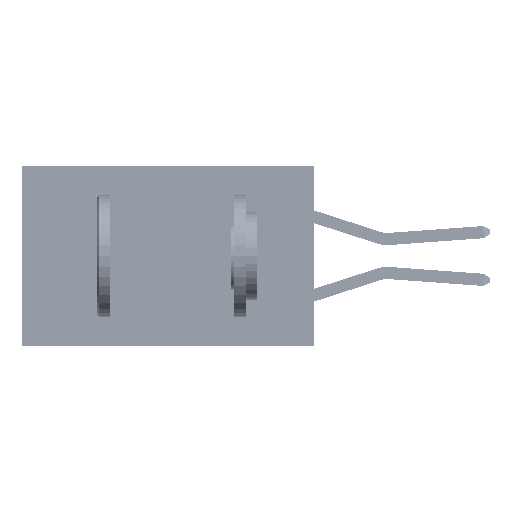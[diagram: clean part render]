
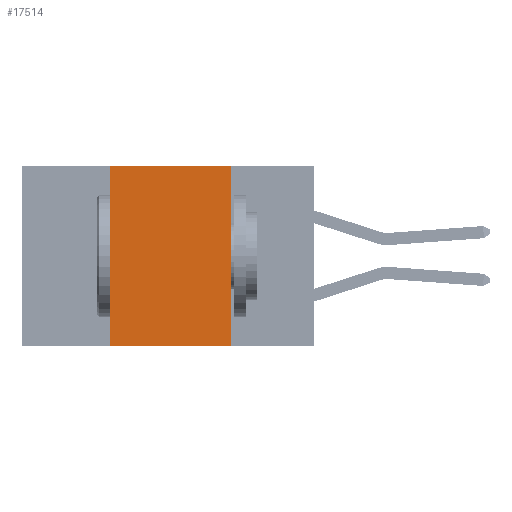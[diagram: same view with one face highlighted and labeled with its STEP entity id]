
A CAD part, left-side view. The second image highlights one B-rep face of the part: STEP entity #17514.
In plain terms, the highlighted planar face has unit normal (-1, 0, 0).
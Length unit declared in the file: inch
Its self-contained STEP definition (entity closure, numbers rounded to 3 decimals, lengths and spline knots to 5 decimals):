
#2994 = VERTEX_POINT ( 'NONE', #39221 ) ;
#3120 = CARTESIAN_POINT ( 'NONE',  ( 0., 0.42, 0. ) ) ;
#3988 = ORIENTED_EDGE ( 'NONE', *, *, #10687, .F. ) ;
#4960 = VERTEX_POINT ( 'NONE', #11925 ) ;
#8691 = EDGE_LOOP ( 'NONE', ( #48236, #26833, #3988, #29303 ) ) ;
#10092 = EDGE_CURVE ( 'NONE', #31452, #2994, #28479, .T. ) ;
#10687 = EDGE_CURVE ( 'NONE', #31452, #4960, #23612, .T. ) ;
#11925 = CARTESIAN_POINT ( 'NONE',  ( 0., 0.42, 0. ) ) ;
#12574 = LINE ( 'NONE', #23094, #21765 ) ;
#13145 = DIRECTION ( 'NONE',  ( 1., 0., 0. ) ) ;
#17514 = ADVANCED_FACE ( 'NONE', ( #49856 ), #32469, .F. ) ;
#18030 = EDGE_CURVE ( 'NONE', #4960, #30088, #28951, .T. ) ;
#18558 = VECTOR ( 'NONE', #28494, 39.37008 ) ;
#18847 = AXIS2_PLACEMENT_3D ( 'NONE', #36596, #13145, #40510 ) ;
#19148 = DIRECTION ( 'NONE',  ( 0., 0., -1. ) ) ;
#21765 = VECTOR ( 'NONE', #19148, 39.37008 ) ;
#23094 = CARTESIAN_POINT ( 'NONE',  ( 0., 0.17, 0. ) ) ;
#23612 = LINE ( 'NONE', #3120, #46233 ) ;
#26801 = DIRECTION ( 'NONE',  ( 0., 0., 1. ) ) ;
#26833 = ORIENTED_EDGE ( 'NONE', *, *, #18030, .F. ) ;
#27071 = CARTESIAN_POINT ( 'NONE',  ( 0., 0.42, -0.37 ) ) ;
#28479 = LINE ( 'NONE', #30786, #36450 ) ;
#28494 = DIRECTION ( 'NONE',  ( 0., -1., 0. ) ) ;
#28951 = LINE ( 'NONE', #36215, #18558 ) ;
#29192 = CARTESIAN_POINT ( 'NONE',  ( 0., 0.17, 0. ) ) ;
#29303 = ORIENTED_EDGE ( 'NONE', *, *, #10092, .T. ) ;
#30088 = VERTEX_POINT ( 'NONE', #29192 ) ;
#30786 = CARTESIAN_POINT ( 'NONE',  ( 0., 0.6, -0.37 ) ) ;
#31452 = VERTEX_POINT ( 'NONE', #27071 ) ;
#32469 = PLANE ( 'NONE',  #18847 ) ;
#36215 = CARTESIAN_POINT ( 'NONE',  ( 0., 0.6, 0. ) ) ;
#36450 = VECTOR ( 'NONE', #42748, 39.37008 ) ;
#36596 = CARTESIAN_POINT ( 'NONE',  ( 0., 0.6, 0. ) ) ;
#39221 = CARTESIAN_POINT ( 'NONE',  ( 0., 0.17, -0.37 ) ) ;
#40510 = DIRECTION ( 'NONE',  ( 0., 0., -1. ) ) ;
#42595 = EDGE_CURVE ( 'NONE', #30088, #2994, #12574, .T. ) ;
#42748 = DIRECTION ( 'NONE',  ( 0., -1., 0. ) ) ;
#46233 = VECTOR ( 'NONE', #26801, 39.37008 ) ;
#48236 = ORIENTED_EDGE ( 'NONE', *, *, #42595, .F. ) ;
#49856 = FACE_OUTER_BOUND ( 'NONE', #8691, .T. ) ;
